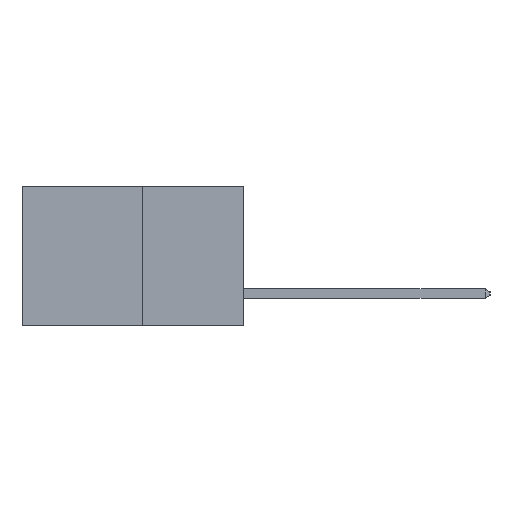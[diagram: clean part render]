
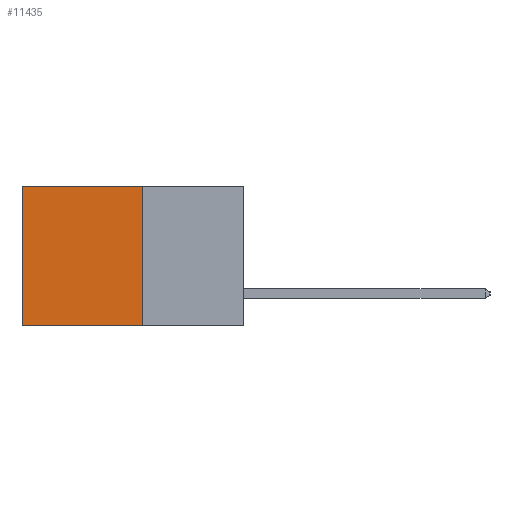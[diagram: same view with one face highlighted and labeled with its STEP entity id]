
A CAD part, left-side view. The second image highlights one B-rep face of the part: STEP entity #11435.
In plain terms, the highlighted planar face has unit normal (-1, 0, 0).
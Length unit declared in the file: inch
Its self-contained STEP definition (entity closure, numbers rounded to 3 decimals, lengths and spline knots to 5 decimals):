
#43 = VERTEX_POINT ( 'NONE', #2432 ) ;
#879 = DIRECTION ( 'NONE',  ( 1., 0., 0. ) ) ;
#1523 = VECTOR ( 'NONE', #3348, 39.37008 ) ;
#1563 = CARTESIAN_POINT ( 'NONE',  ( 0.277, 0.27, -0.37 ) ) ;
#1932 = CARTESIAN_POINT ( 'NONE',  ( 0.277, 0.27, 0. ) ) ;
#2076 = DIRECTION ( 'NONE',  ( 0., 0., -1. ) ) ;
#2096 = CARTESIAN_POINT ( 'NONE',  ( 0.277, 0.59, -0.37 ) ) ;
#2191 = VERTEX_POINT ( 'NONE', #1563 ) ;
#2231 = EDGE_CURVE ( 'NONE', #9895, #9736, #4545, .T. ) ;
#2432 = CARTESIAN_POINT ( 'NONE',  ( 0.277, 0.59, -0.37 ) ) ;
#2673 = CARTESIAN_POINT ( 'NONE',  ( 0.277, 0.59, 0. ) ) ;
#2757 = EDGE_CURVE ( 'NONE', #2191, #43, #11651, .T. ) ;
#3240 = EDGE_LOOP ( 'NONE', ( #12715, #10516, #4146, #6904 ) ) ;
#3348 = DIRECTION ( 'NONE',  ( 0., 1., 0. ) ) ;
#3442 = CARTESIAN_POINT ( 'NONE',  ( 0.277, 0.27, -0.37 ) ) ;
#4034 = EDGE_CURVE ( 'NONE', #9736, #43, #7737, .T. ) ;
#4146 = ORIENTED_EDGE ( 'NONE', *, *, #9201, .F. ) ;
#4466 = LINE ( 'NONE', #8643, #7076 ) ;
#4545 = LINE ( 'NONE', #7150, #7170 ) ;
#5911 = PLANE ( 'NONE',  #12655 ) ;
#6828 = FACE_OUTER_BOUND ( 'NONE', #3240, .T. ) ;
#6904 = ORIENTED_EDGE ( 'NONE', *, *, #2231, .T. ) ;
#7076 = VECTOR ( 'NONE', #9651, 39.37008 ) ;
#7105 = DIRECTION ( 'NONE',  ( 0., 1., 0. ) ) ;
#7150 = CARTESIAN_POINT ( 'NONE',  ( 0.277, 0.27, 0. ) ) ;
#7170 = VECTOR ( 'NONE', #7105, 39.37008 ) ;
#7737 = LINE ( 'NONE', #2096, #12487 ) ;
#7892 = DIRECTION ( 'NONE',  ( 0., 0., -1. ) ) ;
#8643 = CARTESIAN_POINT ( 'NONE',  ( 0.277, 0.27, -0.37 ) ) ;
#9201 = EDGE_CURVE ( 'NONE', #9895, #2191, #4466, .T. ) ;
#9651 = DIRECTION ( 'NONE',  ( 0., 0., -1. ) ) ;
#9736 = VERTEX_POINT ( 'NONE', #2673 ) ;
#9895 = VERTEX_POINT ( 'NONE', #1932 ) ;
#10516 = ORIENTED_EDGE ( 'NONE', *, *, #2757, .F. ) ;
#11435 = ADVANCED_FACE ( 'NONE', ( #6828 ), #5911, .F. ) ;
#11651 = LINE ( 'NONE', #3442, #1523 ) ;
#12487 = VECTOR ( 'NONE', #2076, 39.37008 ) ;
#12611 = CARTESIAN_POINT ( 'NONE',  ( 0.277, 0.27, -0.37 ) ) ;
#12655 = AXIS2_PLACEMENT_3D ( 'NONE', #12611, #879, #7892 ) ;
#12715 = ORIENTED_EDGE ( 'NONE', *, *, #4034, .T. ) ;
